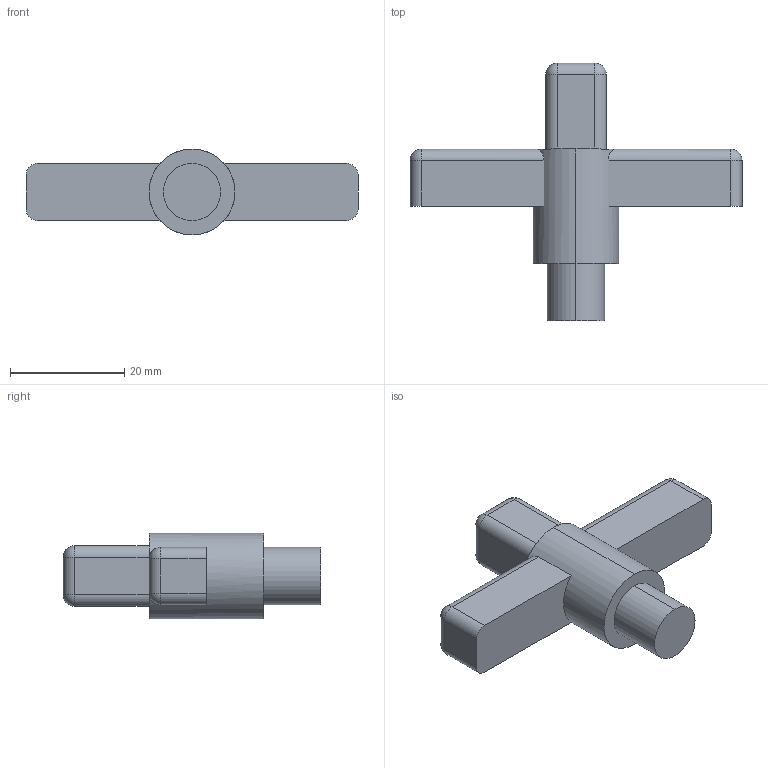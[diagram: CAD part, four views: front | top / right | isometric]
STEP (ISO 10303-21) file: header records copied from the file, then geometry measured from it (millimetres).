
FILE_DESCRIPTION (( 'STEP AP203' ), '1' );
FILE_NAME ('key.STEP', '2013-09-09T02:54:21', ( '' ), ( '' ), 'SwSTEP 2.0', 'SolidWorks 2013', '' );
FILE_SCHEMA (( 'CONFIG_CONTROL_DESIGN' ));
Length unit declared in the file: millimetre
Products named in the file (1): key
Bounding box: 58 x 45 x 15 mm (x, y, z)
Volume: 10219.3 mm3; surface area: 3827 mm2
Topology: 1 solids, 1 shells, 46 faces, 110 edges, 60 vertices
Faces by surface type: cylinder 22, plane 16, sphere 8
Entity records: 1383 total; most frequent: CARTESIAN_POINT 265, DIRECTION 236, ORIENTED_EDGE 204, EDGE_CURVE 102, AXIS2_PLACEMENT_3D 91, VERTEX_POINT 60, VECTOR 54, LINE 54
